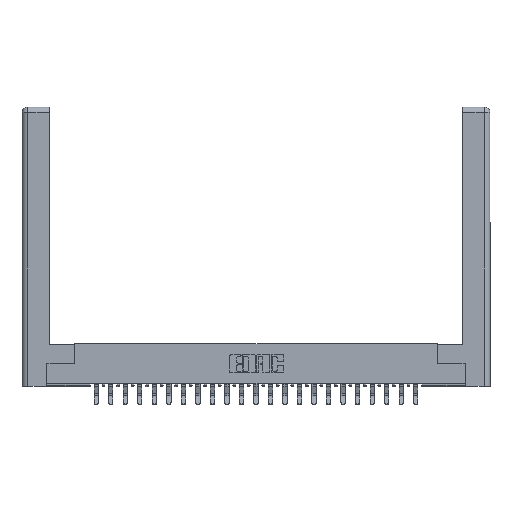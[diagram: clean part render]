
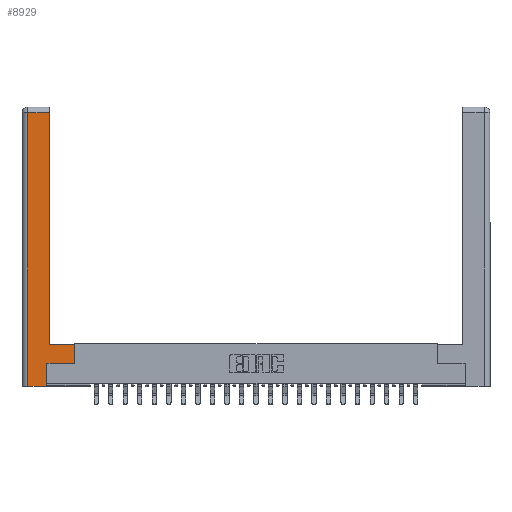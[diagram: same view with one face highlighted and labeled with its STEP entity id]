
A CAD part, top view. The second image highlights one B-rep face of the part: STEP entity #8929.
In plain terms, the highlighted planar face has unit normal (0, 0, 1).
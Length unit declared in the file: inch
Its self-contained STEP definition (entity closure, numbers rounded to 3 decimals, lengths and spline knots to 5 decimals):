
#312 = EDGE_LOOP ( 'NONE', ( #578, #20557, #15016, #16539, #4400, #15034, #20976, #20984 ) ) ;
#476 = EDGE_CURVE ( 'NONE', #25307, #22221, #2542, .T. ) ;
#578 = ORIENTED_EDGE ( 'NONE', *, *, #23817, .T. ) ;
#868 = DIRECTION ( 'NONE',  ( 0., -1., 0. ) ) ;
#1360 = VECTOR ( 'NONE', #20534, 39.37008 ) ;
#1543 = PLANE ( 'NONE',  #23793 ) ;
#2542 = LINE ( 'NONE', #24861, #23199 ) ;
#3847 = CARTESIAN_POINT ( 'NONE',  ( 0., 0., 0. ) ) ;
#4184 = EDGE_CURVE ( 'NONE', #28731, #27824, #20860, .T. ) ;
#4242 = VECTOR ( 'NONE', #21420, 39.37008 ) ;
#4294 = CARTESIAN_POINT ( 'NONE',  ( 0.565, 0.245, 0. ) ) ;
#4400 = ORIENTED_EDGE ( 'NONE', *, *, #476, .T. ) ;
#6171 = DIRECTION ( 'NONE',  ( -1., 0., 0. ) ) ;
#7048 = CARTESIAN_POINT ( 'NONE',  ( 0.265, 0., 0. ) ) ;
#7301 = CARTESIAN_POINT ( 'NONE',  ( 0.295, 3., 0. ) ) ;
#7672 = CARTESIAN_POINT ( 'NONE',  ( 0.265, 0., 0. ) ) ;
#8929 = ADVANCED_FACE ( 'NONE', ( #10739 ), #1543, .F. ) ;
#9206 = CARTESIAN_POINT ( 'NONE',  ( 0.295, 0.45, 0. ) ) ;
#9758 = CARTESIAN_POINT ( 'NONE',  ( 0.0615, 0., 0. ) ) ;
#9797 = VERTEX_POINT ( 'NONE', #12268 ) ;
#10401 = DIRECTION ( 'NONE',  ( 0., 1., 0. ) ) ;
#10739 = FACE_OUTER_BOUND ( 'NONE', #312, .T. ) ;
#12268 = CARTESIAN_POINT ( 'NONE',  ( 0.295, 0.45, 0. ) ) ;
#13257 = LINE ( 'NONE', #9758, #24873 ) ;
#13365 = CARTESIAN_POINT ( 'NONE',  ( 0.0615, 2.94, 0. ) ) ;
#14023 = LINE ( 'NONE', #7301, #4242 ) ;
#14198 = EDGE_CURVE ( 'NONE', #22221, #28731, #18020, .T. ) ;
#14697 = LINE ( 'NONE', #9206, #28860 ) ;
#15016 = ORIENTED_EDGE ( 'NONE', *, *, #21647, .T. ) ;
#15034 = ORIENTED_EDGE ( 'NONE', *, *, #14198, .T. ) ;
#15739 = VERTEX_POINT ( 'NONE', #22567 ) ;
#16539 = ORIENTED_EDGE ( 'NONE', *, *, #28494, .T. ) ;
#17012 = CARTESIAN_POINT ( 'NONE',  ( 0.565, 0.45, 0. ) ) ;
#17270 = CARTESIAN_POINT ( 'NONE',  ( 0.0615, 2.94, 0. ) ) ;
#18020 = LINE ( 'NONE', #4294, #1360 ) ;
#20092 = DIRECTION ( 'NONE',  ( 0., 0., -1. ) ) ;
#20155 = VECTOR ( 'NONE', #10401, 39.37008 ) ;
#20396 = DIRECTION ( 'NONE',  ( -1., 0., 0. ) ) ;
#20534 = DIRECTION ( 'NONE',  ( 1., 0., 0. ) ) ;
#20557 = ORIENTED_EDGE ( 'NONE', *, *, #22082, .T. ) ;
#20860 = LINE ( 'NONE', #17012, #20155 ) ;
#20976 = ORIENTED_EDGE ( 'NONE', *, *, #4184, .T. ) ;
#20984 = ORIENTED_EDGE ( 'NONE', *, *, #24927, .T. ) ;
#21401 = LINE ( 'NONE', #7672, #22832 ) ;
#21420 = DIRECTION ( 'NONE',  ( 0., 1., 0. ) ) ;
#21647 = EDGE_CURVE ( 'NONE', #21766, #15739, #13257, .T. ) ;
#21671 = VERTEX_POINT ( 'NONE', #28626 ) ;
#21675 = CARTESIAN_POINT ( 'NONE',  ( 0.565, 0.45, 0. ) ) ;
#21766 = VERTEX_POINT ( 'NONE', #17270 ) ;
#22082 = EDGE_CURVE ( 'NONE', #21671, #21766, #24467, .T. ) ;
#22221 = VERTEX_POINT ( 'NONE', #25426 ) ;
#22567 = CARTESIAN_POINT ( 'NONE',  ( 0.0615, 0., 0. ) ) ;
#22832 = VECTOR ( 'NONE', #23900, 39.37008 ) ;
#23199 = VECTOR ( 'NONE', #25058, 39.37008 ) ;
#23793 = AXIS2_PLACEMENT_3D ( 'NONE', #3847, #20092, #6171 ) ;
#23817 = EDGE_CURVE ( 'NONE', #9797, #21671, #14023, .T. ) ;
#23900 = DIRECTION ( 'NONE',  ( 1., 0., 0. ) ) ;
#24467 = LINE ( 'NONE', #13365, #29592 ) ;
#24861 = CARTESIAN_POINT ( 'NONE',  ( 0.265, 0.245, 0. ) ) ;
#24873 = VECTOR ( 'NONE', #868, 39.37008 ) ;
#24927 = EDGE_CURVE ( 'NONE', #27824, #9797, #14697, .T. ) ;
#25058 = DIRECTION ( 'NONE',  ( 0., 1., 0. ) ) ;
#25307 = VERTEX_POINT ( 'NONE', #7048 ) ;
#25426 = CARTESIAN_POINT ( 'NONE',  ( 0.265, 0.245, 0. ) ) ;
#27064 = DIRECTION ( 'NONE',  ( -1., 0., 0. ) ) ;
#27824 = VERTEX_POINT ( 'NONE', #21675 ) ;
#28348 = CARTESIAN_POINT ( 'NONE',  ( 0.565, 0.245, 0. ) ) ;
#28494 = EDGE_CURVE ( 'NONE', #15739, #25307, #21401, .T. ) ;
#28626 = CARTESIAN_POINT ( 'NONE',  ( 0.295, 2.94, 0. ) ) ;
#28731 = VERTEX_POINT ( 'NONE', #28348 ) ;
#28860 = VECTOR ( 'NONE', #20396, 39.37008 ) ;
#29592 = VECTOR ( 'NONE', #27064, 39.37008 ) ;
